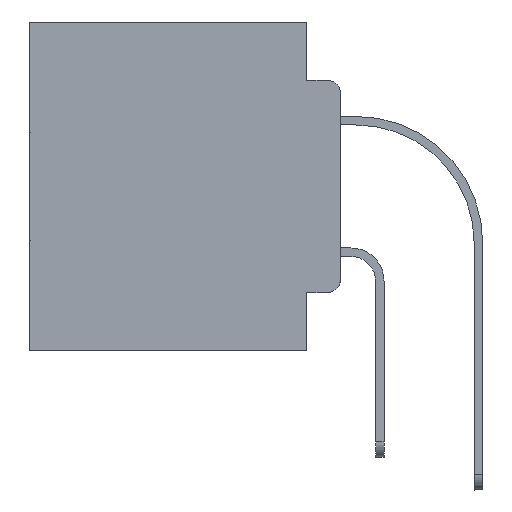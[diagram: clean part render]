
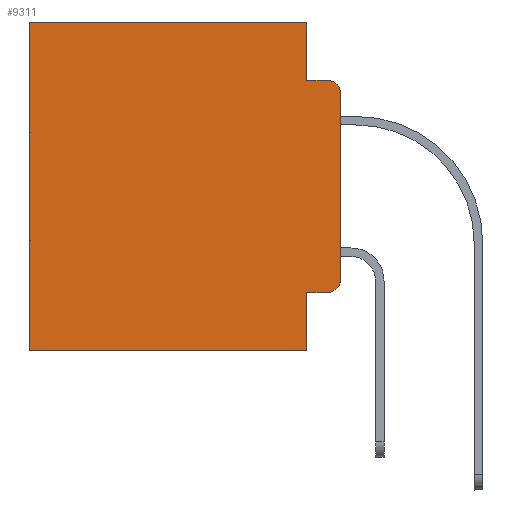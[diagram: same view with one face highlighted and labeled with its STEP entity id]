
A CAD part, left-side view. The second image highlights one B-rep face of the part: STEP entity #9311.
In plain terms, the highlighted planar face has unit normal (-1, 0, 0).
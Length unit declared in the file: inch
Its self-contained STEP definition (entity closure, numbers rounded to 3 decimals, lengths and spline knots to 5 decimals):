
#63 = VERTEX_POINT ( 'NONE', #2722 ) ;
#650 = CARTESIAN_POINT ( 'NONE',  ( 0.298, 0.051, 0. ) ) ;
#757 = DIRECTION ( 'NONE',  ( -1., 0., 0. ) ) ;
#832 = DIRECTION ( 'NONE',  ( 0., -1., 0. ) ) ;
#849 = EDGE_CURVE ( 'NONE', #31655, #17077, #11139, .T. ) ;
#1798 = EDGE_CURVE ( 'NONE', #6765, #17077, #13855, .T. ) ;
#2063 = EDGE_CURVE ( 'NONE', #63, #7216, #27581, .T. ) ;
#2286 = CARTESIAN_POINT ( 'NONE',  ( 0.298, 0., -0.3915 ) ) ;
#2382 = VECTOR ( 'NONE', #15398, 39.37008 ) ;
#2722 = CARTESIAN_POINT ( 'NONE',  ( 0.298, 0.051, -0.0885 ) ) ;
#3102 = VERTEX_POINT ( 'NONE', #14769 ) ;
#3116 = ORIENTED_EDGE ( 'NONE', *, *, #849, .F. ) ;
#3292 = EDGE_LOOP ( 'NONE', ( #8161, #15060, #19331, #20203, #16217, #22712, #3116, #17857, #10232, #10979 ) ) ;
#3558 = CARTESIAN_POINT ( 'NONE',  ( 0.298, 0.02, -0.3915 ) ) ;
#3728 = LINE ( 'NONE', #4049, #12616 ) ;
#3870 = LINE ( 'NONE', #31416, #22552 ) ;
#4049 = CARTESIAN_POINT ( 'NONE',  ( 0.298, 0.051, 0. ) ) ;
#5139 = EDGE_CURVE ( 'NONE', #30048, #6765, #3870, .T. ) ;
#5613 = AXIS2_PLACEMENT_3D ( 'NONE', #3558, #757, #16043 ) ;
#6765 = VERTEX_POINT ( 'NONE', #17545 ) ;
#7216 = VERTEX_POINT ( 'NONE', #10624 ) ;
#7534 = DIRECTION ( 'NONE',  ( 0., 0., -1. ) ) ;
#7616 = AXIS2_PLACEMENT_3D ( 'NONE', #15257, #20495, #7534 ) ;
#7927 = CARTESIAN_POINT ( 'NONE',  ( 0.298, 0., 0. ) ) ;
#8129 = CIRCLE ( 'NONE', #7616, 0.02 ) ;
#8161 = ORIENTED_EDGE ( 'NONE', *, *, #22462, .F. ) ;
#8328 = VECTOR ( 'NONE', #832, 39.37008 ) ;
#8625 = DIRECTION ( 'NONE',  ( 0., 1., 0. ) ) ;
#8679 = EDGE_CURVE ( 'NONE', #30048, #63, #3728, .T. ) ;
#9311 = ADVANCED_FACE ( 'NONE', ( #20250 ), #22868, .F. ) ;
#10126 = VECTOR ( 'NONE', #13309, 39.37008 ) ;
#10232 = ORIENTED_EDGE ( 'NONE', *, *, #28884, .T. ) ;
#10304 = LINE ( 'NONE', #20315, #2382 ) ;
#10396 = DIRECTION ( 'NONE',  ( 0., 0., -1. ) ) ;
#10624 = CARTESIAN_POINT ( 'NONE',  ( 0.298, 0.02, -0.0885 ) ) ;
#10686 = CARTESIAN_POINT ( 'NONE',  ( 0.298, 0., 0. ) ) ;
#10979 = ORIENTED_EDGE ( 'NONE', *, *, #30231, .T. ) ;
#11139 = LINE ( 'NONE', #23114, #12446 ) ;
#12446 = VECTOR ( 'NONE', #20659, 39.37008 ) ;
#12616 = VECTOR ( 'NONE', #28656, 39.37008 ) ;
#12829 = CARTESIAN_POINT ( 'NONE',  ( 0.298, 0.473, -0.5 ) ) ;
#13000 = DIRECTION ( 'NONE',  ( 0., 0., -1. ) ) ;
#13305 = AXIS2_PLACEMENT_3D ( 'NONE', #7927, #15334, #10396 ) ;
#13309 = DIRECTION ( 'NONE',  ( 0., 0., -1. ) ) ;
#13855 = LINE ( 'NONE', #26123, #15693 ) ;
#14769 = CARTESIAN_POINT ( 'NONE',  ( 0.298, 0.02, -0.4115 ) ) ;
#15060 = ORIENTED_EDGE ( 'NONE', *, *, #17515, .T. ) ;
#15257 = CARTESIAN_POINT ( 'NONE',  ( 0.298, 0.02, -0.1085 ) ) ;
#15334 = DIRECTION ( 'NONE',  ( 1., 0., 0. ) ) ;
#15398 = DIRECTION ( 'NONE',  ( 0., -1., 0. ) ) ;
#15693 = VECTOR ( 'NONE', #29237, 39.37008 ) ;
#15785 = CARTESIAN_POINT ( 'NONE',  ( 0.298, 0.051, -0.0885 ) ) ;
#15797 = VECTOR ( 'NONE', #13000, 39.37008 ) ;
#16043 = DIRECTION ( 'NONE',  ( 0., 0., -1. ) ) ;
#16217 = ORIENTED_EDGE ( 'NONE', *, *, #5139, .T. ) ;
#17077 = VERTEX_POINT ( 'NONE', #12829 ) ;
#17384 = CARTESIAN_POINT ( 'NONE',  ( 0.298, 0.051, 0. ) ) ;
#17515 = EDGE_CURVE ( 'NONE', #27144, #7216, #8129, .T. ) ;
#17545 = CARTESIAN_POINT ( 'NONE',  ( 0.298, 0.473, 0. ) ) ;
#17857 = ORIENTED_EDGE ( 'NONE', *, *, #24470, .F. ) ;
#19331 = ORIENTED_EDGE ( 'NONE', *, *, #2063, .F. ) ;
#19764 = CIRCLE ( 'NONE', #5613, 0.02 ) ;
#20203 = ORIENTED_EDGE ( 'NONE', *, *, #8679, .F. ) ;
#20250 = FACE_OUTER_BOUND ( 'NONE', #3292, .T. ) ;
#20315 = CARTESIAN_POINT ( 'NONE',  ( 0.298, 0.051, -0.4115 ) ) ;
#20495 = DIRECTION ( 'NONE',  ( -1., 0., 0. ) ) ;
#20659 = DIRECTION ( 'NONE',  ( 0., 1., 0. ) ) ;
#22462 = EDGE_CURVE ( 'NONE', #27144, #28238, #28062, .T. ) ;
#22552 = VECTOR ( 'NONE', #8625, 39.37008 ) ;
#22712 = ORIENTED_EDGE ( 'NONE', *, *, #1798, .T. ) ;
#22868 = PLANE ( 'NONE',  #13305 ) ;
#23114 = CARTESIAN_POINT ( 'NONE',  ( 0.298, 0., -0.5 ) ) ;
#23138 = LINE ( 'NONE', #650, #10126 ) ;
#24470 = EDGE_CURVE ( 'NONE', #25686, #31655, #23138, .T. ) ;
#24792 = CARTESIAN_POINT ( 'NONE',  ( 0.298, 0., -0.1085 ) ) ;
#25686 = VERTEX_POINT ( 'NONE', #27400 ) ;
#26123 = CARTESIAN_POINT ( 'NONE',  ( 0.298, 0.473, 0. ) ) ;
#27144 = VERTEX_POINT ( 'NONE', #24792 ) ;
#27310 = CARTESIAN_POINT ( 'NONE',  ( 0.298, 0.051, -0.5 ) ) ;
#27400 = CARTESIAN_POINT ( 'NONE',  ( 0.298, 0.051, -0.4115 ) ) ;
#27581 = LINE ( 'NONE', #15785, #8328 ) ;
#28062 = LINE ( 'NONE', #10686, #15797 ) ;
#28238 = VERTEX_POINT ( 'NONE', #2286 ) ;
#28656 = DIRECTION ( 'NONE',  ( 0., 0., -1. ) ) ;
#28884 = EDGE_CURVE ( 'NONE', #25686, #3102, #10304, .T. ) ;
#29237 = DIRECTION ( 'NONE',  ( 0., 0., -1. ) ) ;
#30048 = VERTEX_POINT ( 'NONE', #17384 ) ;
#30231 = EDGE_CURVE ( 'NONE', #3102, #28238, #19764, .T. ) ;
#31416 = CARTESIAN_POINT ( 'NONE',  ( 0.298, 0., 0. ) ) ;
#31655 = VERTEX_POINT ( 'NONE', #27310 ) ;
